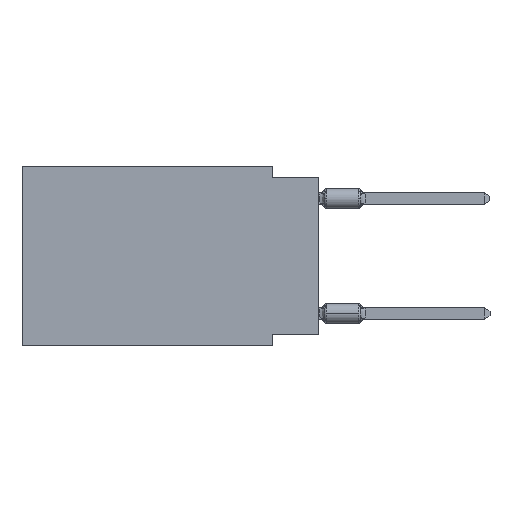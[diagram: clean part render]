
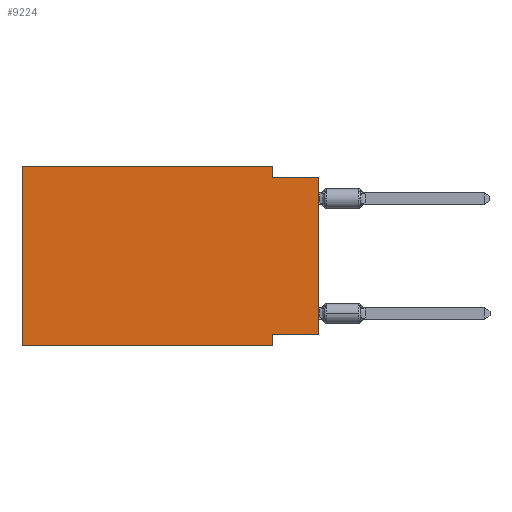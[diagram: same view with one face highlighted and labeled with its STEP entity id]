
A CAD part, left-side view. The second image highlights one B-rep face of the part: STEP entity #9224.
In plain terms, the highlighted planar face has unit normal (-1, 0, 0).
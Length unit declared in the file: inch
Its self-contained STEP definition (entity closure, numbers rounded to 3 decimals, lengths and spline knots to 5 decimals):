
#272 = EDGE_CURVE ( 'NONE', #9762, #5034, #7564, .T. ) ;
#308 = CARTESIAN_POINT ( 'NONE',  ( 0., 0.645, 0. ) ) ;
#339 = CARTESIAN_POINT ( 'NONE',  ( 0., 0., -0.025 ) ) ;
#448 = DIRECTION ( 'NONE',  ( 0., -1., 0. ) ) ;
#715 = CARTESIAN_POINT ( 'NONE',  ( 0., 0.1, -0.39 ) ) ;
#912 = CARTESIAN_POINT ( 'NONE',  ( 0., 0.645, 0. ) ) ;
#916 = EDGE_CURVE ( 'NONE', #19793, #13427, #13125, .T. ) ;
#1043 = CARTESIAN_POINT ( 'NONE',  ( 0., 0.1, 0. ) ) ;
#1417 = VECTOR ( 'NONE', #16376, 39.37008 ) ;
#1925 = LINE ( 'NONE', #308, #5789 ) ;
#2485 = DIRECTION ( 'NONE',  ( 0., -1., 0. ) ) ;
#2623 = ORIENTED_EDGE ( 'NONE', *, *, #6946, .F. ) ;
#3378 = ORIENTED_EDGE ( 'NONE', *, *, #916, .T. ) ;
#3495 = LINE ( 'NONE', #10564, #19482 ) ;
#3534 = DIRECTION ( 'NONE',  ( 0., 0., 1. ) ) ;
#3892 = VERTEX_POINT ( 'NONE', #8015 ) ;
#4040 = LINE ( 'NONE', #715, #12132 ) ;
#4199 = VERTEX_POINT ( 'NONE', #20561 ) ;
#4332 = PLANE ( 'NONE',  #14775 ) ;
#4484 = ORIENTED_EDGE ( 'NONE', *, *, #4998, .F. ) ;
#4853 = CARTESIAN_POINT ( 'NONE',  ( 0., 0.1, -0.365 ) ) ;
#4893 = VECTOR ( 'NONE', #19018, 39.37008 ) ;
#4998 = EDGE_CURVE ( 'NONE', #16946, #16673, #4040, .T. ) ;
#5034 = VERTEX_POINT ( 'NONE', #1043 ) ;
#5789 = VECTOR ( 'NONE', #3534, 39.37008 ) ;
#6009 = VECTOR ( 'NONE', #19289, 39.37008 ) ;
#6946 = EDGE_CURVE ( 'NONE', #4199, #9762, #1925, .T. ) ;
#7239 = ORIENTED_EDGE ( 'NONE', *, *, #16365, .T. ) ;
#7420 = LINE ( 'NONE', #20404, #4893 ) ;
#7462 = CARTESIAN_POINT ( 'NONE',  ( 0., 0.645, 0. ) ) ;
#7564 = LINE ( 'NONE', #7462, #15212 ) ;
#8015 = CARTESIAN_POINT ( 'NONE',  ( 0., 0.1, -0.025 ) ) ;
#8287 = EDGE_CURVE ( 'NONE', #3892, #13427, #18410, .T. ) ;
#9099 = EDGE_LOOP ( 'NONE', ( #3378, #21274, #20546, #13521, #2623, #7239, #4484, #19852 ) ) ;
#9224 = ADVANCED_FACE ( 'NONE', ( #17776 ), #4332, .F. ) ;
#9762 = VERTEX_POINT ( 'NONE', #14582 ) ;
#9979 = CARTESIAN_POINT ( 'NONE',  ( 0., 0., -0.365 ) ) ;
#10564 = CARTESIAN_POINT ( 'NONE',  ( 0., 0., -0.365 ) ) ;
#10990 = CARTESIAN_POINT ( 'NONE',  ( 0., 0.1, 0. ) ) ;
#12057 = DIRECTION ( 'NONE',  ( 0., 1., 0. ) ) ;
#12132 = VECTOR ( 'NONE', #17487, 39.37008 ) ;
#12592 = DIRECTION ( 'NONE',  ( 1., 0., 0. ) ) ;
#13125 = LINE ( 'NONE', #19836, #1417 ) ;
#13427 = VERTEX_POINT ( 'NONE', #19352 ) ;
#13521 = ORIENTED_EDGE ( 'NONE', *, *, #272, .F. ) ;
#14582 = CARTESIAN_POINT ( 'NONE',  ( 0., 0.645, 0. ) ) ;
#14775 = AXIS2_PLACEMENT_3D ( 'NONE', #912, #12592, #17459 ) ;
#15212 = VECTOR ( 'NONE', #2485, 39.37008 ) ;
#15938 = LINE ( 'NONE', #10990, #6009 ) ;
#16365 = EDGE_CURVE ( 'NONE', #4199, #16673, #7420, .T. ) ;
#16376 = DIRECTION ( 'NONE',  ( 0., 0., 1. ) ) ;
#16673 = VERTEX_POINT ( 'NONE', #16720 ) ;
#16720 = CARTESIAN_POINT ( 'NONE',  ( 0., 0.1, -0.39 ) ) ;
#16946 = VERTEX_POINT ( 'NONE', #4853 ) ;
#17233 = VECTOR ( 'NONE', #448, 39.37008 ) ;
#17459 = DIRECTION ( 'NONE',  ( 0., 0., -1. ) ) ;
#17487 = DIRECTION ( 'NONE',  ( 0., 0., -1. ) ) ;
#17776 = FACE_OUTER_BOUND ( 'NONE', #9099, .T. ) ;
#18210 = EDGE_CURVE ( 'NONE', #19793, #16946, #3495, .T. ) ;
#18358 = EDGE_CURVE ( 'NONE', #5034, #3892, #15938, .T. ) ;
#18410 = LINE ( 'NONE', #339, #17233 ) ;
#19018 = DIRECTION ( 'NONE',  ( 0., -1., 0. ) ) ;
#19289 = DIRECTION ( 'NONE',  ( 0., 0., -1. ) ) ;
#19352 = CARTESIAN_POINT ( 'NONE',  ( 0., 0., -0.025 ) ) ;
#19482 = VECTOR ( 'NONE', #12057, 39.37008 ) ;
#19793 = VERTEX_POINT ( 'NONE', #9979 ) ;
#19836 = CARTESIAN_POINT ( 'NONE',  ( 0., 0., 0. ) ) ;
#19852 = ORIENTED_EDGE ( 'NONE', *, *, #18210, .F. ) ;
#20404 = CARTESIAN_POINT ( 'NONE',  ( 0., 0.645, -0.39 ) ) ;
#20546 = ORIENTED_EDGE ( 'NONE', *, *, #18358, .F. ) ;
#20561 = CARTESIAN_POINT ( 'NONE',  ( 0., 0.645, -0.39 ) ) ;
#21274 = ORIENTED_EDGE ( 'NONE', *, *, #8287, .F. ) ;
